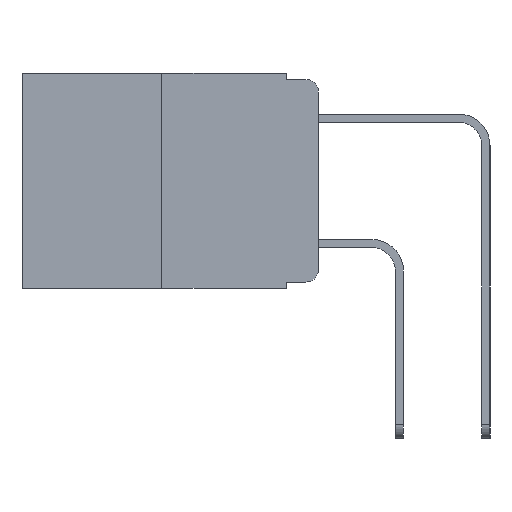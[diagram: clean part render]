
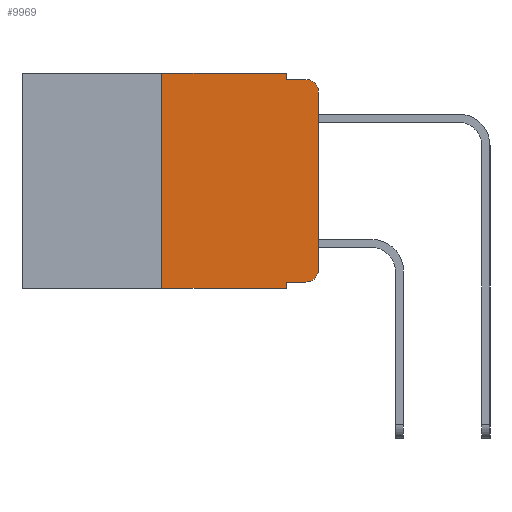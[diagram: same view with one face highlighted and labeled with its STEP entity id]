
A CAD part, left-side view. The second image highlights one B-rep face of the part: STEP entity #9969.
In plain terms, the highlighted planar face has unit normal (-1, 0, 0).
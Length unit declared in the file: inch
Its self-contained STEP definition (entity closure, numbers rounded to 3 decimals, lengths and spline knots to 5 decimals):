
#416 = DIRECTION ( 'NONE',  ( 1., 0., 0. ) ) ;
#468 = FACE_OUTER_BOUND ( 'NONE', #13664, .T. ) ;
#784 = CARTESIAN_POINT ( 'NONE',  ( 0., 0.02, -0.333 ) ) ;
#1310 = VECTOR ( 'NONE', #11443, 39.37008 ) ;
#1493 = EDGE_CURVE ( 'NONE', #14354, #12194, #5355, .T. ) ;
#1628 = VERTEX_POINT ( 'NONE', #13628 ) ;
#2545 = DIRECTION ( 'NONE',  ( 0., -1., 0. ) ) ;
#2737 = VECTOR ( 'NONE', #10693, 39.37008 ) ;
#2785 = EDGE_CURVE ( 'NONE', #16245, #6527, #7814, .T. ) ;
#3724 = ORIENTED_EDGE ( 'NONE', *, *, #16396, .T. ) ;
#3751 = CARTESIAN_POINT ( 'NONE',  ( 0., 0.02, -0.313 ) ) ;
#3874 = VECTOR ( 'NONE', #7849, 39.37008 ) ;
#3980 = AXIS2_PLACEMENT_3D ( 'NONE', #15919, #5620, #17617 ) ;
#4908 = EDGE_CURVE ( 'NONE', #14354, #11261, #10967, .T. ) ;
#5355 = LINE ( 'NONE', #13249, #21746 ) ;
#5458 = DIRECTION ( 'NONE',  ( 0., 0., -1. ) ) ;
#5474 = CARTESIAN_POINT ( 'NONE',  ( 0., 0.473, 0. ) ) ;
#5620 = DIRECTION ( 'NONE',  ( -1., 0., 0. ) ) ;
#5773 = CARTESIAN_POINT ( 'NONE',  ( 0., 0.473, -0.343 ) ) ;
#6038 = EDGE_CURVE ( 'NONE', #1628, #16245, #10655, .T. ) ;
#6048 = DIRECTION ( 'NONE',  ( 0., 0., -1. ) ) ;
#6270 = VECTOR ( 'NONE', #10992, 39.37008 ) ;
#6527 = VERTEX_POINT ( 'NONE', #11263 ) ;
#7814 = LINE ( 'NONE', #15629, #2737 ) ;
#7849 = DIRECTION ( 'NONE',  ( 0., 0., 1. ) ) ;
#8008 = DIRECTION ( 'NONE',  ( 0., -1., 0. ) ) ;
#8121 = LINE ( 'NONE', #14569, #21069 ) ;
#8347 = EDGE_CURVE ( 'NONE', #6527, #14384, #8902, .T. ) ;
#8419 = ORIENTED_EDGE ( 'NONE', *, *, #12142, .T. ) ;
#8781 = AXIS2_PLACEMENT_3D ( 'NONE', #5474, #416, #12437 ) ;
#8902 = LINE ( 'NONE', #18021, #9457 ) ;
#9156 = ORIENTED_EDGE ( 'NONE', *, *, #15281, .F. ) ;
#9457 = VECTOR ( 'NONE', #6048, 39.37008 ) ;
#9929 = VERTEX_POINT ( 'NONE', #15714 ) ;
#9969 = ADVANCED_FACE ( 'NONE', ( #468 ), #20749, .F. ) ;
#9993 = DIRECTION ( 'NONE',  ( 0., 0., 1. ) ) ;
#10655 = LINE ( 'NONE', #18452, #14171 ) ;
#10693 = DIRECTION ( 'NONE',  ( 0., -1., 0. ) ) ;
#10709 = CARTESIAN_POINT ( 'NONE',  ( 0., 0.051, -0.343 ) ) ;
#10874 = LINE ( 'NONE', #5773, #6270 ) ;
#10967 = LINE ( 'NONE', #19805, #1310 ) ;
#10992 = DIRECTION ( 'NONE',  ( 0., -1., 0. ) ) ;
#11261 = VERTEX_POINT ( 'NONE', #10709 ) ;
#11263 = CARTESIAN_POINT ( 'NONE',  ( 0., 0.051, 0. ) ) ;
#11443 = DIRECTION ( 'NONE',  ( 0., 0., -1. ) ) ;
#11668 = ORIENTED_EDGE ( 'NONE', *, *, #19692, .T. ) ;
#11962 = CARTESIAN_POINT ( 'NONE',  ( 0., 0.051, -0.333 ) ) ;
#12142 = EDGE_CURVE ( 'NONE', #1628, #11261, #10874, .T. ) ;
#12194 = VERTEX_POINT ( 'NONE', #784 ) ;
#12437 = DIRECTION ( 'NONE',  ( 0., 0., -1. ) ) ;
#12940 = ORIENTED_EDGE ( 'NONE', *, *, #8347, .F. ) ;
#13042 = LINE ( 'NONE', #18139, #3874 ) ;
#13058 = ORIENTED_EDGE ( 'NONE', *, *, #6038, .F. ) ;
#13249 = CARTESIAN_POINT ( 'NONE',  ( 0., 0.051, -0.333 ) ) ;
#13296 = ORIENTED_EDGE ( 'NONE', *, *, #2785, .F. ) ;
#13612 = AXIS2_PLACEMENT_3D ( 'NONE', #3751, #15763, #5458 ) ;
#13628 = CARTESIAN_POINT ( 'NONE',  ( 0., 0.25, -0.343 ) ) ;
#13664 = EDGE_LOOP ( 'NONE', ( #11668, #3724, #9156, #12940, #13296, #13058, #8419, #14118, #18408, #14934 ) ) ;
#14118 = ORIENTED_EDGE ( 'NONE', *, *, #4908, .F. ) ;
#14171 = VECTOR ( 'NONE', #9993, 39.37008 ) ;
#14354 = VERTEX_POINT ( 'NONE', #11962 ) ;
#14384 = VERTEX_POINT ( 'NONE', #20443 ) ;
#14569 = CARTESIAN_POINT ( 'NONE',  ( 0., 0.051, -0.01 ) ) ;
#14934 = ORIENTED_EDGE ( 'NONE', *, *, #21216, .T. ) ;
#15281 = EDGE_CURVE ( 'NONE', #14384, #18536, #8121, .T. ) ;
#15629 = CARTESIAN_POINT ( 'NONE',  ( 0., 0.473, 0. ) ) ;
#15714 = CARTESIAN_POINT ( 'NONE',  ( 0., 0., -0.313 ) ) ;
#15763 = DIRECTION ( 'NONE',  ( -1., 0., 0. ) ) ;
#15919 = CARTESIAN_POINT ( 'NONE',  ( 0., 0.02, -0.03 ) ) ;
#16245 = VERTEX_POINT ( 'NONE', #20459 ) ;
#16396 = EDGE_CURVE ( 'NONE', #18612, #18536, #16911, .T. ) ;
#16911 = CIRCLE ( 'NONE', #3980, 0.02 ) ;
#16934 = CARTESIAN_POINT ( 'NONE',  ( 0., 0., -0.03 ) ) ;
#17617 = DIRECTION ( 'NONE',  ( 0., 0., -1. ) ) ;
#17718 = CIRCLE ( 'NONE', #13612, 0.02 ) ;
#18021 = CARTESIAN_POINT ( 'NONE',  ( 0., 0.051, 0. ) ) ;
#18139 = CARTESIAN_POINT ( 'NONE',  ( 0., 0., 0. ) ) ;
#18408 = ORIENTED_EDGE ( 'NONE', *, *, #1493, .T. ) ;
#18452 = CARTESIAN_POINT ( 'NONE',  ( 0., 0.25, 0. ) ) ;
#18536 = VERTEX_POINT ( 'NONE', #20012 ) ;
#18612 = VERTEX_POINT ( 'NONE', #16934 ) ;
#19692 = EDGE_CURVE ( 'NONE', #9929, #18612, #13042, .T. ) ;
#19805 = CARTESIAN_POINT ( 'NONE',  ( 0., 0.051, 0. ) ) ;
#20012 = CARTESIAN_POINT ( 'NONE',  ( 0., 0.02, -0.01 ) ) ;
#20443 = CARTESIAN_POINT ( 'NONE',  ( 0., 0.051, -0.01 ) ) ;
#20459 = CARTESIAN_POINT ( 'NONE',  ( 0., 0.25, 0. ) ) ;
#20749 = PLANE ( 'NONE',  #8781 ) ;
#21069 = VECTOR ( 'NONE', #2545, 39.37008 ) ;
#21216 = EDGE_CURVE ( 'NONE', #12194, #9929, #17718, .T. ) ;
#21746 = VECTOR ( 'NONE', #8008, 39.37008 ) ;
